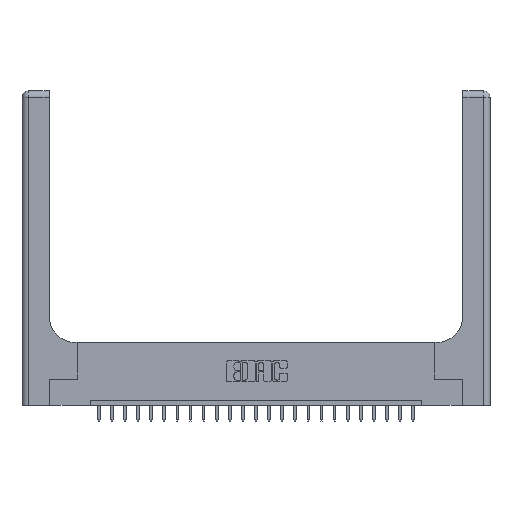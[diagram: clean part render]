
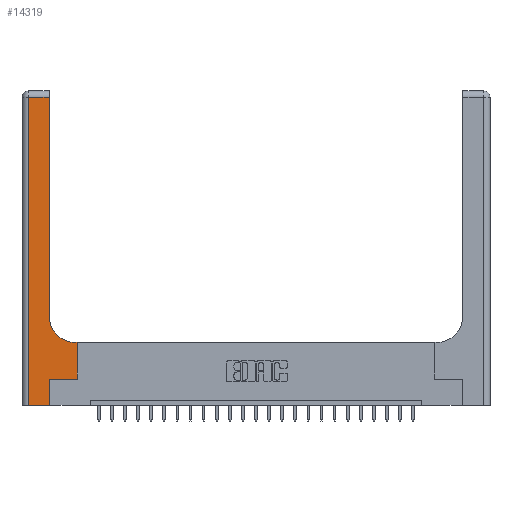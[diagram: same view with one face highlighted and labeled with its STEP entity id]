
A CAD part, top view. The second image highlights one B-rep face of the part: STEP entity #14319.
In plain terms, the highlighted planar face has unit normal (0, 0, 1).
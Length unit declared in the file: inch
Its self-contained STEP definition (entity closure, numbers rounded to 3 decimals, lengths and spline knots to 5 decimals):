
#1168 = CARTESIAN_POINT ( 'NONE',  ( 0.528, 0.25, 0.37 ) ) ;
#1348 = DIRECTION ( 'NONE',  ( 0., 1., 0. ) ) ;
#1374 = ORIENTED_EDGE ( 'NONE', *, *, #2135, .T. ) ;
#1821 = DIRECTION ( 'NONE',  ( 0., 0., -1. ) ) ;
#1852 = EDGE_CURVE ( 'NONE', #7086, #20952, #10461, .T. ) ;
#1870 = VERTEX_POINT ( 'NONE', #19578 ) ;
#2135 = EDGE_CURVE ( 'NONE', #20952, #4175, #18728, .T. ) ;
#2472 = CARTESIAN_POINT ( 'NONE',  ( 0.265, 0., 0.37 ) ) ;
#2710 = DIRECTION ( 'NONE',  ( -1., 0., 0. ) ) ;
#2872 = EDGE_CURVE ( 'NONE', #18852, #15736, #8972, .T. ) ;
#3017 = VECTOR ( 'NONE', #20706, 39.37008 ) ;
#3599 = LINE ( 'NONE', #8823, #13932 ) ;
#3703 = CIRCLE ( 'NONE', #6727, 0.25 ) ;
#3714 = FACE_OUTER_BOUND ( 'NONE', #17130, .T. ) ;
#3829 = DIRECTION ( 'NONE',  ( -1., 0., 0. ) ) ;
#4175 = VERTEX_POINT ( 'NONE', #19031 ) ;
#4213 = VECTOR ( 'NONE', #18999, 39.37008 ) ;
#5375 = CARTESIAN_POINT ( 'NONE',  ( 0., 3., 0.37 ) ) ;
#5679 = ORIENTED_EDGE ( 'NONE', *, *, #7487, .T. ) ;
#5974 = ORIENTED_EDGE ( 'NONE', *, *, #9077, .T. ) ;
#6014 = EDGE_CURVE ( 'NONE', #4175, #18852, #3703, .T. ) ;
#6492 = VERTEX_POINT ( 'NONE', #20510 ) ;
#6727 = AXIS2_PLACEMENT_3D ( 'NONE', #18526, #12965, #16277 ) ;
#6741 = VECTOR ( 'NONE', #19102, 39.37008 ) ;
#6888 = VERTEX_POINT ( 'NONE', #16118 ) ;
#7009 = ORIENTED_EDGE ( 'NONE', *, *, #6014, .T. ) ;
#7086 = VERTEX_POINT ( 'NONE', #1168 ) ;
#7150 = DIRECTION ( 'NONE',  ( 0., -1., 0. ) ) ;
#7487 = EDGE_CURVE ( 'NONE', #6888, #6492, #3599, .T. ) ;
#8316 = DIRECTION ( 'NONE',  ( -1., 0., 0. ) ) ;
#8757 = ORIENTED_EDGE ( 'NONE', *, *, #16486, .T. ) ;
#8823 = CARTESIAN_POINT ( 'NONE',  ( 0.06, 3., 0.37 ) ) ;
#8870 = ORIENTED_EDGE ( 'NONE', *, *, #23039, .T. ) ;
#8972 = LINE ( 'NONE', #17108, #4213 ) ;
#9077 = EDGE_CURVE ( 'NONE', #6492, #19087, #14765, .T. ) ;
#9303 = VECTOR ( 'NONE', #23173, 39.37008 ) ;
#9483 = VECTOR ( 'NONE', #8316, 39.37008 ) ;
#9816 = LINE ( 'NONE', #22490, #15671 ) ;
#10461 = LINE ( 'NONE', #17570, #16645 ) ;
#11616 = ORIENTED_EDGE ( 'NONE', *, *, #1852, .T. ) ;
#11634 = CARTESIAN_POINT ( 'NONE',  ( 0.26, 0.85, 0.37 ) ) ;
#12043 = EDGE_CURVE ( 'NONE', #1870, #7086, #15942, .T. ) ;
#12464 = ORIENTED_EDGE ( 'NONE', *, *, #2872, .T. ) ;
#12939 = CARTESIAN_POINT ( 'NONE',  ( 0.265, 0.25, 0.37 ) ) ;
#12965 = DIRECTION ( 'NONE',  ( 0., 0., -1. ) ) ;
#13485 = LINE ( 'NONE', #2472, #3017 ) ;
#13932 = VECTOR ( 'NONE', #7150, 39.37008 ) ;
#14319 = ADVANCED_FACE ( 'NONE', ( #3714 ), #21604, .F. ) ;
#14765 = LINE ( 'NONE', #21977, #6741 ) ;
#15073 = CARTESIAN_POINT ( 'NONE',  ( 0.26, 0.6, 0.37 ) ) ;
#15671 = VECTOR ( 'NONE', #2710, 39.37008 ) ;
#15736 = VERTEX_POINT ( 'NONE', #18863 ) ;
#15942 = LINE ( 'NONE', #12939, #9303 ) ;
#16118 = CARTESIAN_POINT ( 'NONE',  ( 0.06, 2.94, 0.37 ) ) ;
#16277 = DIRECTION ( 'NONE',  ( 1., 0., 0. ) ) ;
#16486 = EDGE_CURVE ( 'NONE', #19087, #1870, #13485, .T. ) ;
#16645 = VECTOR ( 'NONE', #1348, 39.37008 ) ;
#16933 = ORIENTED_EDGE ( 'NONE', *, *, #12043, .T. ) ;
#17108 = CARTESIAN_POINT ( 'NONE',  ( 0.26, 3., 0.37 ) ) ;
#17130 = EDGE_LOOP ( 'NONE', ( #12464, #8870, #5679, #5974, #8757, #16933, #11616, #1374, #7009 ) ) ;
#17570 = CARTESIAN_POINT ( 'NONE',  ( 0.528, 0.25, 0.37 ) ) ;
#18437 = AXIS2_PLACEMENT_3D ( 'NONE', #5375, #1821, #3829 ) ;
#18526 = CARTESIAN_POINT ( 'NONE',  ( 0.51, 0.85, 0.37 ) ) ;
#18542 = CARTESIAN_POINT ( 'NONE',  ( 0.265, 0., 0.37 ) ) ;
#18728 = LINE ( 'NONE', #15073, #9483 ) ;
#18852 = VERTEX_POINT ( 'NONE', #11634 ) ;
#18863 = CARTESIAN_POINT ( 'NONE',  ( 0.26, 2.94, 0.37 ) ) ;
#18999 = DIRECTION ( 'NONE',  ( 0., 1., 0. ) ) ;
#19031 = CARTESIAN_POINT ( 'NONE',  ( 0.51, 0.6, 0.37 ) ) ;
#19087 = VERTEX_POINT ( 'NONE', #18542 ) ;
#19102 = DIRECTION ( 'NONE',  ( 1., 0., 0. ) ) ;
#19578 = CARTESIAN_POINT ( 'NONE',  ( 0.265, 0.25, 0.37 ) ) ;
#20510 = CARTESIAN_POINT ( 'NONE',  ( 0.06, 0., 0.37 ) ) ;
#20706 = DIRECTION ( 'NONE',  ( 0., 1., 0. ) ) ;
#20952 = VERTEX_POINT ( 'NONE', #21489 ) ;
#21489 = CARTESIAN_POINT ( 'NONE',  ( 0.528, 0.6, 0.37 ) ) ;
#21604 = PLANE ( 'NONE',  #18437 ) ;
#21977 = CARTESIAN_POINT ( 'NONE',  ( 0., 0., 0.37 ) ) ;
#22490 = CARTESIAN_POINT ( 'NONE',  ( 0., 2.94, 0.37 ) ) ;
#23039 = EDGE_CURVE ( 'NONE', #15736, #6888, #9816, .T. ) ;
#23173 = DIRECTION ( 'NONE',  ( 1., 0., 0. ) ) ;
